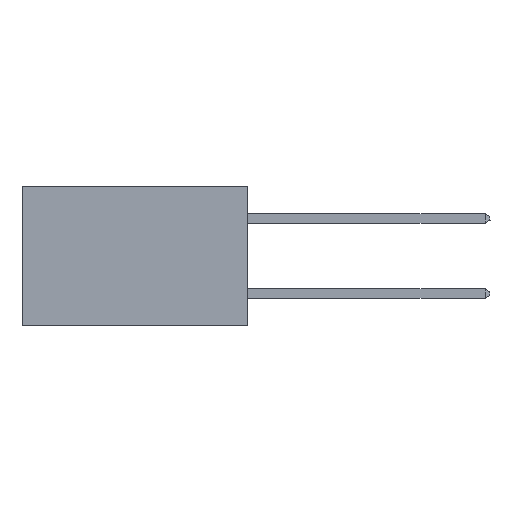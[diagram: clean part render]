
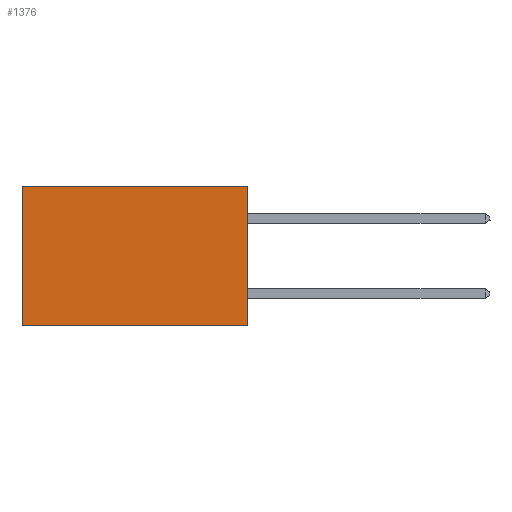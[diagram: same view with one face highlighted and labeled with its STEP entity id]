
A CAD part, left-side view. The second image highlights one B-rep face of the part: STEP entity #1376.
In plain terms, the highlighted planar face has unit normal (-1, 0, 0).
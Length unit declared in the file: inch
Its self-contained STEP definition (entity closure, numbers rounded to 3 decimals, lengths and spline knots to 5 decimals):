
#784 = VERTEX_POINT ( 'NONE', #19721 ) ;
#1376 = ADVANCED_FACE ( 'NONE', ( #8972 ), #21821, .F. ) ;
#1437 = CARTESIAN_POINT ( 'NONE',  ( 0.298, 0.6, 0. ) ) ;
#1746 = DIRECTION ( 'NONE',  ( 0., 0., -1. ) ) ;
#3128 = ORIENTED_EDGE ( 'NONE', *, *, #25575, .F. ) ;
#3519 = DIRECTION ( 'NONE',  ( 0., 0., -1. ) ) ;
#3554 = DIRECTION ( 'NONE',  ( 0., 1., 0. ) ) ;
#3597 = VERTEX_POINT ( 'NONE', #23657 ) ;
#4310 = VECTOR ( 'NONE', #3519, 39.37008 ) ;
#6872 = ORIENTED_EDGE ( 'NONE', *, *, #20264, .F. ) ;
#8388 = CARTESIAN_POINT ( 'NONE',  ( 0.298, 0., 0. ) ) ;
#8972 = FACE_OUTER_BOUND ( 'NONE', #17308, .T. ) ;
#9964 = AXIS2_PLACEMENT_3D ( 'NONE', #29225, #14497, #17257 ) ;
#11735 = VERTEX_POINT ( 'NONE', #21966 ) ;
#11899 = LINE ( 'NONE', #1437, #22549 ) ;
#13388 = CARTESIAN_POINT ( 'NONE',  ( 0.298, 0., 0. ) ) ;
#14497 = DIRECTION ( 'NONE',  ( 1., 0., 0. ) ) ;
#16383 = VERTEX_POINT ( 'NONE', #19669 ) ;
#16544 = DIRECTION ( 'NONE',  ( 0., 1., 0. ) ) ;
#17257 = DIRECTION ( 'NONE',  ( 0., 0., -1. ) ) ;
#17308 = EDGE_LOOP ( 'NONE', ( #17385, #6872, #3128, #19138 ) ) ;
#17385 = ORIENTED_EDGE ( 'NONE', *, *, #20728, .T. ) ;
#18032 = VECTOR ( 'NONE', #16544, 39.37008 ) ;
#19138 = ORIENTED_EDGE ( 'NONE', *, *, #23731, .T. ) ;
#19351 = LINE ( 'NONE', #8388, #27363 ) ;
#19669 = CARTESIAN_POINT ( 'NONE',  ( 0.298, 0., 0. ) ) ;
#19721 = CARTESIAN_POINT ( 'NONE',  ( 0.298, 0., -0.37 ) ) ;
#20264 = EDGE_CURVE ( 'NONE', #784, #11735, #27939, .T. ) ;
#20728 = EDGE_CURVE ( 'NONE', #3597, #11735, #11899, .T. ) ;
#21821 = PLANE ( 'NONE',  #9964 ) ;
#21966 = CARTESIAN_POINT ( 'NONE',  ( 0.298, 0.6, -0.37 ) ) ;
#22549 = VECTOR ( 'NONE', #1746, 39.37008 ) ;
#23657 = CARTESIAN_POINT ( 'NONE',  ( 0.298, 0.6, 0. ) ) ;
#23731 = EDGE_CURVE ( 'NONE', #16383, #3597, #19351, .T. ) ;
#25575 = EDGE_CURVE ( 'NONE', #16383, #784, #28386, .T. ) ;
#26437 = CARTESIAN_POINT ( 'NONE',  ( 0.298, 0., -0.37 ) ) ;
#27363 = VECTOR ( 'NONE', #3554, 39.37008 ) ;
#27939 = LINE ( 'NONE', #26437, #18032 ) ;
#28386 = LINE ( 'NONE', #13388, #4310 ) ;
#29225 = CARTESIAN_POINT ( 'NONE',  ( 0.298, 0., 0. ) ) ;
